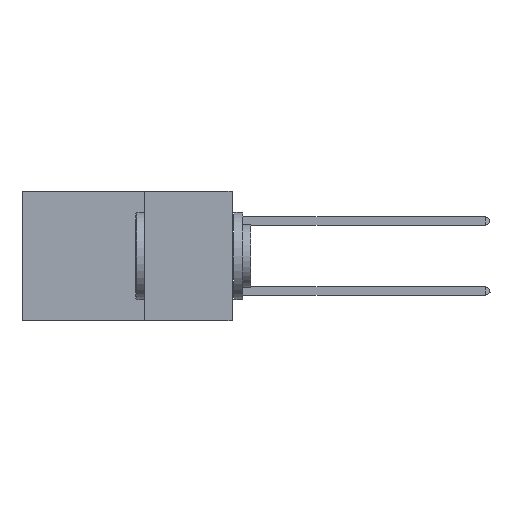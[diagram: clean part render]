
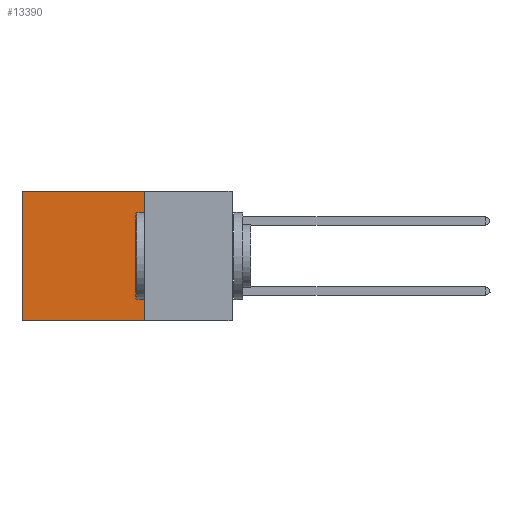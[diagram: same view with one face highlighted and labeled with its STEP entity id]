
A CAD part, left-side view. The second image highlights one B-rep face of the part: STEP entity #13390.
In plain terms, the highlighted planar face has unit normal (-1, 0, 0).
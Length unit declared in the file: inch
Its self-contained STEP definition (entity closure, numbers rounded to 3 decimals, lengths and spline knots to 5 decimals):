
#161 = EDGE_CURVE ( 'NONE', #15436, #5242, #1369, .T. ) ;
#384 = VERTEX_POINT ( 'NONE', #14629 ) ;
#793 = VECTOR ( 'NONE', #3952, 39.37008 ) ;
#978 = VECTOR ( 'NONE', #15535, 39.37008 ) ;
#1369 = LINE ( 'NONE', #5028, #978 ) ;
#2740 = EDGE_LOOP ( 'NONE', ( #13446, #16620, #4170, #14736 ) ) ;
#2747 = DIRECTION ( 'NONE',  ( 0., 0., -1. ) ) ;
#3952 = DIRECTION ( 'NONE',  ( 0., 1., 0. ) ) ;
#4170 = ORIENTED_EDGE ( 'NONE', *, *, #14422, .F. ) ;
#4245 = LINE ( 'NONE', #13603, #15762 ) ;
#4248 = LINE ( 'NONE', #7580, #793 ) ;
#5028 = CARTESIAN_POINT ( 'NONE',  ( 0.2875, 0.25, 0. ) ) ;
#5242 = VERTEX_POINT ( 'NONE', #7302 ) ;
#5551 = EDGE_CURVE ( 'NONE', #5242, #384, #4245, .T. ) ;
#5841 = CARTESIAN_POINT ( 'NONE',  ( 0.2875, 0.25, 0. ) ) ;
#5924 = CARTESIAN_POINT ( 'NONE',  ( 0.2875, 0.25, 0. ) ) ;
#6462 = LINE ( 'NONE', #5841, #14111 ) ;
#7038 = DIRECTION ( 'NONE',  ( 0., 0., -1. ) ) ;
#7302 = CARTESIAN_POINT ( 'NONE',  ( 0.2875, 0.6, 0. ) ) ;
#7580 = CARTESIAN_POINT ( 'NONE',  ( 0.2875, 0.25, -0.37 ) ) ;
#7932 = CARTESIAN_POINT ( 'NONE',  ( 0.2875, 0.25, 0. ) ) ;
#9547 = CARTESIAN_POINT ( 'NONE',  ( 0.2875, 0.25, -0.37 ) ) ;
#11352 = VERTEX_POINT ( 'NONE', #9547 ) ;
#11775 = DIRECTION ( 'NONE',  ( 1., 0., 0. ) ) ;
#11878 = PLANE ( 'NONE',  #14500 ) ;
#12799 = DIRECTION ( 'NONE',  ( 0., 0., -1. ) ) ;
#13390 = ADVANCED_FACE ( 'NONE', ( #15365 ), #11878, .F. ) ;
#13446 = ORIENTED_EDGE ( 'NONE', *, *, #5551, .T. ) ;
#13603 = CARTESIAN_POINT ( 'NONE',  ( 0.2875, 0.6, 0. ) ) ;
#13817 = EDGE_CURVE ( 'NONE', #11352, #384, #4248, .T. ) ;
#14111 = VECTOR ( 'NONE', #12799, 39.37008 ) ;
#14422 = EDGE_CURVE ( 'NONE', #15436, #11352, #6462, .T. ) ;
#14500 = AXIS2_PLACEMENT_3D ( 'NONE', #7932, #11775, #2747 ) ;
#14629 = CARTESIAN_POINT ( 'NONE',  ( 0.2875, 0.6, -0.37 ) ) ;
#14736 = ORIENTED_EDGE ( 'NONE', *, *, #161, .T. ) ;
#15365 = FACE_OUTER_BOUND ( 'NONE', #2740, .T. ) ;
#15436 = VERTEX_POINT ( 'NONE', #5924 ) ;
#15535 = DIRECTION ( 'NONE',  ( 0., 1., 0. ) ) ;
#15762 = VECTOR ( 'NONE', #7038, 39.37008 ) ;
#16620 = ORIENTED_EDGE ( 'NONE', *, *, #13817, .F. ) ;
